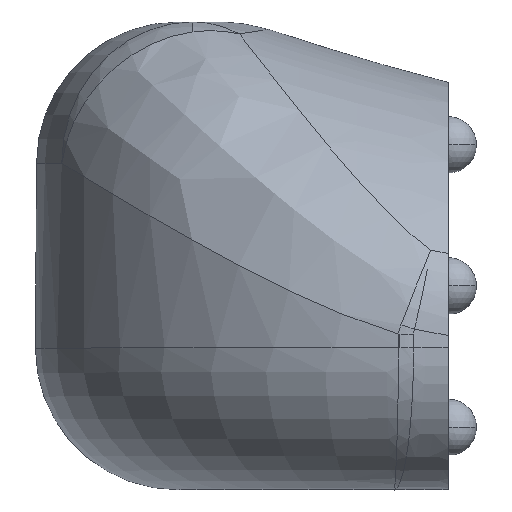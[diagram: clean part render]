
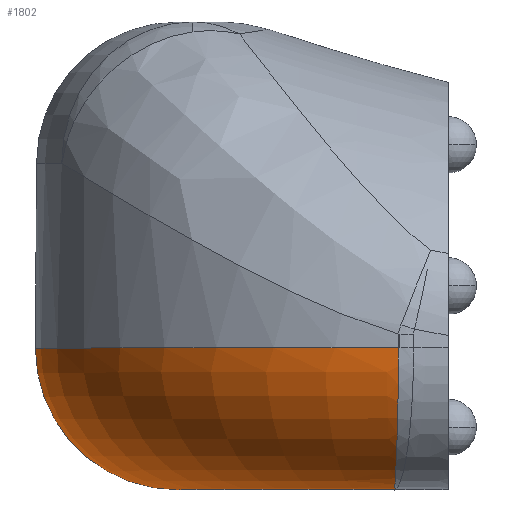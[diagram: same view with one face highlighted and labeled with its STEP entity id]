
A CAD part, top view. The second image highlights one B-rep face of the part: STEP entity #1802.
In plain terms, the highlighted toroidal (fillet/blend) face has major radius 16.269 mm and minor radius 10 mm.
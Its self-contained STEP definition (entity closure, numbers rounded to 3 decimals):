
#4 = CARTESIAN_POINT ( 'NONE',  ( -294.564, -64.049, 4.547 ) ) ;
#122 = CARTESIAN_POINT ( 'NONE',  ( -295.364, -63.414, 24.321 ) ) ;
#143 = VERTEX_POINT ( 'NONE', #1130 ) ;
#253 = ORIENTED_EDGE ( 'NONE', *, *, #685, .F. ) ;
#271 = AXIS2_PLACEMENT_3D ( 'NONE', #1382, #319, #312 ) ;
#288 = CARTESIAN_POINT ( 'NONE',  ( -295.137, -54.049, 30.81 ) ) ;
#312 = DIRECTION ( 'NONE',  ( -1., 0., 0. ) ) ;
#319 = DIRECTION ( 'NONE',  ( 0., 1., 0. ) ) ;
#325 = CARTESIAN_POINT ( 'NONE',  ( -295.151, -56.659, 30.486 ) ) ;
#330 = CARTESIAN_POINT ( 'NONE',  ( -295.16, -57.286, 30.294 ) ) ;
#338 = DIRECTION ( 'NONE',  ( -1., 0., 0. ) ) ;
#349 = DIRECTION ( 'NONE',  ( 0., -1., 0. ) ) ;
#417 = DIRECTION ( 'NONE',  ( 0., 1., 0. ) ) ;
#421 = AXIS2_PLACEMENT_3D ( 'NONE', #4, #349, #338 ) ;
#439 = VERTEX_POINT ( 'NONE', #494 ) ;
#459 = EDGE_CURVE ( 'NONE', #143, #439, #1170, .T. ) ;
#460 = ORIENTED_EDGE ( 'NONE', *, *, #972, .F. ) ;
#465 = CARTESIAN_POINT ( 'NONE',  ( -295.422, -64.049, 20.794 ) ) ;
#484 = DIRECTION ( 'NONE',  ( 0., 0., -1. ) ) ;
#494 = CARTESIAN_POINT ( 'NONE',  ( -295.137, -54.049, 30.81 ) ) ;
#531 = CARTESIAN_POINT ( 'NONE',  ( -295.422, -64.049, 20.794 ) ) ;
#555 = CARTESIAN_POINT ( 'NONE',  ( -294.564, -54.049, 4.547 ) ) ;
#590 = EDGE_CURVE ( 'NONE', #439, #1324, #741, .T. ) ;
#635 = FACE_OUTER_BOUND ( 'NONE', #1155, .T. ) ;
#648 = CARTESIAN_POINT ( 'NONE',  ( -295.391, -63.794, 23.064 ) ) ;
#651 = ORIENTED_EDGE ( 'NONE', *, *, #459, .F. ) ;
#685 = EDGE_CURVE ( 'NONE', #1324, #1075, #780, .T. ) ;
#701 = DIRECTION ( 'NONE',  ( -1., 0., 0. ) ) ;
#741 = B_SPLINE_CURVE_WITH_KNOTS ( 'NONE', 3,
 ( #288, #1699, #1674, #325, #330, #1729, #1709, #1722, #1706, #1750, #1741, #921, #1024, #1116, #1733, #122, #1151, #1788, #648, #1757, #1322, #1065, #1031, #465 ),
 .UNSPECIFIED., .F., .F.,
 ( 4, 2, 2, 2, 2, 2, 2, 2, 2, 2, 2, 4 ),
 ( 0., 0.002, 0.004, 0.005, 0.006, 0.008, 0.01, 0.012, 0.013, 0.014, 0.015, 0.016 ),
 .UNSPECIFIED. ) ;
#780 = CIRCLE ( 'NONE', #421, 16.269 ) ;
#921 = CARTESIAN_POINT ( 'NONE',  ( -295.273, -61.587, 27.409 ) ) ;
#972 = EDGE_CURVE ( 'NONE', #1075, #143, #1517, .T. ) ;
#1014 = TOROIDAL_SURFACE ( 'NONE', #1436, 16.269, 10. ) ;
#1024 = CARTESIAN_POINT ( 'NONE',  ( -295.291, -62.008, 26.893 ) ) ;
#1031 = CARTESIAN_POINT ( 'NONE',  ( -295.419, -64.049, 21.123 ) ) ;
#1065 = CARTESIAN_POINT ( 'NONE',  ( -295.415, -64.033, 21.452 ) ) ;
#1069 = CARTESIAN_POINT ( 'NONE',  ( -310.833, -64.049, 4.547 ) ) ;
#1075 = VERTEX_POINT ( 'NONE', #1069 ) ;
#1116 = CARTESIAN_POINT ( 'NONE',  ( -295.325, -62.732, 25.806 ) ) ;
#1130 = CARTESIAN_POINT ( 'NONE',  ( -320.833, -54.049, 4.547 ) ) ;
#1151 = CARTESIAN_POINT ( 'NONE',  ( -295.371, -63.526, 24.009 ) ) ;
#1155 = EDGE_LOOP ( 'NONE', ( #460, #253, #1384, #651 ) ) ;
#1170 = CIRCLE ( 'NONE', #271, 26.269 ) ;
#1296 = CARTESIAN_POINT ( 'NONE',  ( -310.833, -54.049, 4.547 ) ) ;
#1322 = CARTESIAN_POINT ( 'NONE',  ( -295.407, -63.969, 22.102 ) ) ;
#1324 = VERTEX_POINT ( 'NONE', #531 ) ;
#1382 = CARTESIAN_POINT ( 'NONE',  ( -294.564, -54.049, 4.547 ) ) ;
#1384 = ORIENTED_EDGE ( 'NONE', *, *, #590, .F. ) ;
#1432 = DIRECTION ( 'NONE',  ( -1., 0., 0. ) ) ;
#1436 = AXIS2_PLACEMENT_3D ( 'NONE', #555, #417, #701 ) ;
#1517 = CIRCLE ( 'NONE', #1749, 10. ) ;
#1674 = CARTESIAN_POINT ( 'NONE',  ( -295.14, -55.364, 30.745 ) ) ;
#1699 = CARTESIAN_POINT ( 'NONE',  ( -295.137, -54.71, 30.81 ) ) ;
#1706 = CARTESIAN_POINT ( 'NONE',  ( -295.202, -59.345, 29.297 ) ) ;
#1709 = CARTESIAN_POINT ( 'NONE',  ( -295.182, -58.483, 29.778 ) ) ;
#1722 = CARTESIAN_POINT ( 'NONE',  ( -295.195, -59.06, 29.468 ) ) ;
#1729 = CARTESIAN_POINT ( 'NONE',  ( -295.176, -58.188, 29.918 ) ) ;
#1733 = CARTESIAN_POINT ( 'NONE',  ( -295.341, -63.038, 25.231 ) ) ;
#1741 = CARTESIAN_POINT ( 'NONE',  ( -295.24, -60.665, 28.334 ) ) ;
#1749 = AXIS2_PLACEMENT_3D ( 'NONE', #1296, #484, #1432 ) ;
#1750 = CARTESIAN_POINT ( 'NONE',  ( -295.224, -60.162, 28.748 ) ) ;
#1757 = CARTESIAN_POINT ( 'NONE',  ( -295.402, -63.921, 22.425 ) ) ;
#1788 = CARTESIAN_POINT ( 'NONE',  ( -295.384, -63.715, 23.381 ) ) ;
#1802 = ADVANCED_FACE ( 'NONE', ( #635 ), #1014, .T. ) ;
